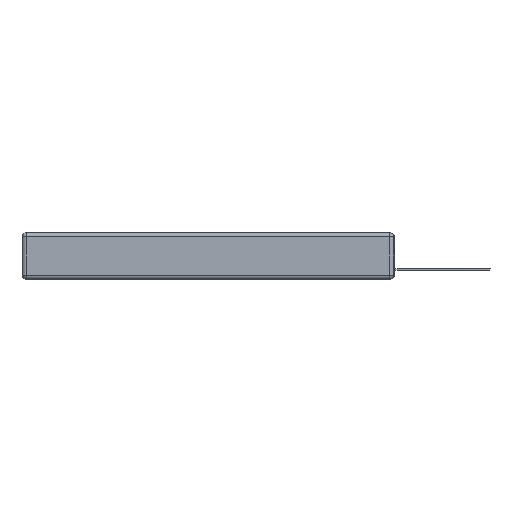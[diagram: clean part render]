
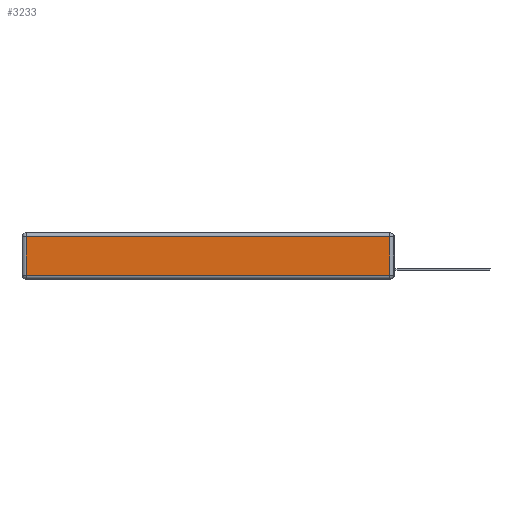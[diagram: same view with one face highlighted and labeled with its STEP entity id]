
A CAD part, left-side view. The second image highlights one B-rep face of the part: STEP entity #3233.
In plain terms, the highlighted planar face has unit normal (-1, 0, 0).
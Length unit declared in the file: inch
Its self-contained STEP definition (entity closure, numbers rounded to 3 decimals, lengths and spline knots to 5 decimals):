
#131 = VECTOR ( 'NONE', #6218, 39.37008 ) ;
#718 = DIRECTION ( 'NONE',  ( -1., 0., 0. ) ) ;
#759 = DIRECTION ( 'NONE',  ( 0., 0., 1. ) ) ;
#1004 = VERTEX_POINT ( 'NONE', #9659 ) ;
#1171 = VERTEX_POINT ( 'NONE', #7440 ) ;
#2163 = LINE ( 'NONE', #10132, #4862 ) ;
#2259 = EDGE_CURVE ( 'NONE', #9111, #11672, #2163, .T. ) ;
#2880 = EDGE_LOOP ( 'NONE', ( #11445, #12951, #11690, #9492 ) ) ;
#2951 = EDGE_CURVE ( 'NONE', #1004, #9111, #10203, .T. ) ;
#3233 = ADVANCED_FACE ( 'NONE', ( #3572 ), #7691, .T. ) ;
#3572 = FACE_OUTER_BOUND ( 'NONE', #2880, .T. ) ;
#3931 = EDGE_CURVE ( 'NONE', #11672, #1171, #9884, .T. ) ;
#4149 = DIRECTION ( 'NONE',  ( 0., 0., -1. ) ) ;
#4862 = VECTOR ( 'NONE', #4149, 39.37008 ) ;
#6218 = DIRECTION ( 'NONE',  ( 0., 1., 0. ) ) ;
#6719 = CARTESIAN_POINT ( 'NONE',  ( 0., 0., -0.343 ) ) ;
#7440 = CARTESIAN_POINT ( 'NONE',  ( 0., 0.03, -0.313 ) ) ;
#7691 = PLANE ( 'NONE',  #8231 ) ;
#8231 = AXIS2_PLACEMENT_3D ( 'NONE', #6719, #718, #759 ) ;
#8784 = CARTESIAN_POINT ( 'NONE',  ( 0., 2.72, -0.313 ) ) ;
#9011 = DIRECTION ( 'NONE',  ( 0., -1., 0. ) ) ;
#9111 = VERTEX_POINT ( 'NONE', #11762 ) ;
#9451 = LINE ( 'NONE', #12681, #11347 ) ;
#9492 = ORIENTED_EDGE ( 'NONE', *, *, #2259, .T. ) ;
#9659 = CARTESIAN_POINT ( 'NONE',  ( 0., 0.03, -0.03 ) ) ;
#9737 = EDGE_CURVE ( 'NONE', #1171, #1004, #9451, .T. ) ;
#9884 = LINE ( 'NONE', #9900, #12257 ) ;
#9900 = CARTESIAN_POINT ( 'NONE',  ( 0., 0., -0.313 ) ) ;
#10132 = CARTESIAN_POINT ( 'NONE',  ( 0., 2.72, -0.343 ) ) ;
#10203 = LINE ( 'NONE', #12280, #131 ) ;
#11347 = VECTOR ( 'NONE', #12637, 39.37008 ) ;
#11445 = ORIENTED_EDGE ( 'NONE', *, *, #3931, .T. ) ;
#11672 = VERTEX_POINT ( 'NONE', #8784 ) ;
#11690 = ORIENTED_EDGE ( 'NONE', *, *, #2951, .T. ) ;
#11762 = CARTESIAN_POINT ( 'NONE',  ( 0., 2.72, -0.03 ) ) ;
#12257 = VECTOR ( 'NONE', #9011, 39.37008 ) ;
#12280 = CARTESIAN_POINT ( 'NONE',  ( 0., 2.75, -0.03 ) ) ;
#12637 = DIRECTION ( 'NONE',  ( 0., 0., 1. ) ) ;
#12681 = CARTESIAN_POINT ( 'NONE',  ( 0., 0.03, -0.343 ) ) ;
#12951 = ORIENTED_EDGE ( 'NONE', *, *, #9737, .T. ) ;
